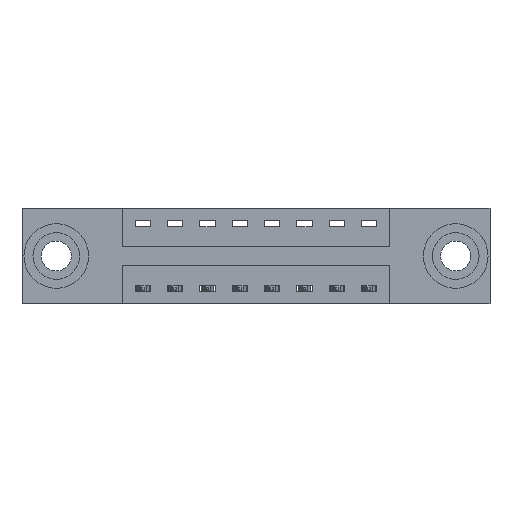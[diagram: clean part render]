
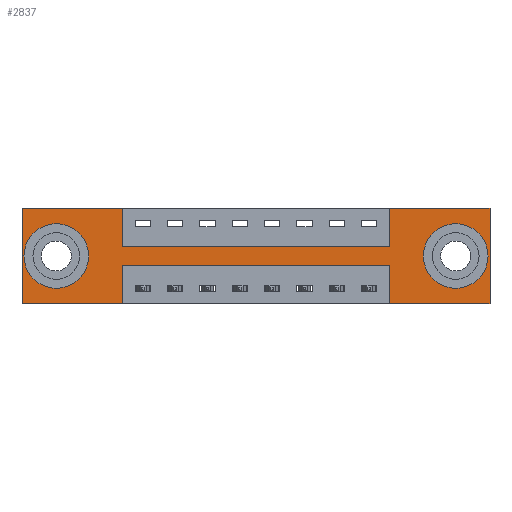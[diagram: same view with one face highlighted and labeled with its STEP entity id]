
A CAD part, front view. The second image highlights one B-rep face of the part: STEP entity #2837.
In plain terms, the highlighted planar face has unit normal (0, -1, 0).
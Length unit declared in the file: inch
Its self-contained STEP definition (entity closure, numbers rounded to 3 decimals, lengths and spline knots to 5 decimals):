
#114 = EDGE_CURVE ( 'NONE', #8169, #7383, #6678, .T. ) ;
#211 = CARTESIAN_POINT ( 'NONE',  ( 0., 0., -0.37 ) ) ;
#252 = LINE ( 'NONE', #2517, #8794 ) ;
#321 = CARTESIAN_POINT ( 'NONE',  ( 0.1325, 0., -0.185 ) ) ;
#346 = ORIENTED_EDGE ( 'NONE', *, *, #6904, .F. ) ;
#357 = CARTESIAN_POINT ( 'NONE',  ( 0., 0., -0.37 ) ) ;
#386 = CARTESIAN_POINT ( 'NONE',  ( 0., 0., 0. ) ) ;
#388 = ORIENTED_EDGE ( 'NONE', *, *, #9088, .F. ) ;
#441 = VERTEX_POINT ( 'NONE', #493 ) ;
#476 = VERTEX_POINT ( 'NONE', #3159 ) ;
#493 = CARTESIAN_POINT ( 'NONE',  ( 0.3875, 0., -0.37 ) ) ;
#588 = VECTOR ( 'NONE', #3738, 39.37008 ) ;
#693 = CARTESIAN_POINT ( 'NONE',  ( 0.3875, 0., -0.15 ) ) ;
#766 = CARTESIAN_POINT ( 'NONE',  ( 0., 0., 0. ) ) ;
#890 = CARTESIAN_POINT ( 'NONE',  ( 0.3875, 0., 0. ) ) ;
#983 = CARTESIAN_POINT ( 'NONE',  ( 0., 0., 0. ) ) ;
#1047 = DIRECTION ( 'NONE',  ( 0., 1., 0. ) ) ;
#1128 = VERTEX_POINT ( 'NONE', #7396 ) ;
#1168 = LINE ( 'NONE', #6201, #8599 ) ;
#1303 = AXIS2_PLACEMENT_3D ( 'NONE', #3767, #10361, #6446 ) ;
#1441 = EDGE_CURVE ( 'NONE', #8724, #7299, #5891, .T. ) ;
#1520 = ORIENTED_EDGE ( 'NONE', *, *, #4039, .F. ) ;
#1630 = DIRECTION ( 'NONE',  ( 1., 0., 0. ) ) ;
#1701 = VERTEX_POINT ( 'NONE', #5114 ) ;
#1726 = FACE_BOUND ( 'NONE', #5411, .T. ) ;
#1796 = EDGE_CURVE ( 'NONE', #476, #1128, #1168, .T. ) ;
#1880 = CARTESIAN_POINT ( 'NONE',  ( 1.4225, 0., -0.37 ) ) ;
#1891 = DIRECTION ( 'NONE',  ( 0., 0., -1. ) ) ;
#2003 = ORIENTED_EDGE ( 'NONE', *, *, #10641, .F. ) ;
#2126 = CARTESIAN_POINT ( 'NONE',  ( 0., 0., -0.37 ) ) ;
#2240 = EDGE_CURVE ( 'NONE', #7383, #8169, #3048, .T. ) ;
#2427 = ORIENTED_EDGE ( 'NONE', *, *, #6433, .F. ) ;
#2454 = CARTESIAN_POINT ( 'NONE',  ( 1.4225, 0., -0.37 ) ) ;
#2517 = CARTESIAN_POINT ( 'NONE',  ( 1.81, 0., 0. ) ) ;
#2661 = VERTEX_POINT ( 'NONE', #8579 ) ;
#2837 = ADVANCED_FACE ( 'NONE', ( #3336, #1726, #5143 ), #7646, .T. ) ;
#2914 = VERTEX_POINT ( 'NONE', #4494 ) ;
#2925 = CARTESIAN_POINT ( 'NONE',  ( 1.81, 0., -0.37 ) ) ;
#2957 = VECTOR ( 'NONE', #4897, 39.37008 ) ;
#3048 = CIRCLE ( 'NONE', #3399, 0.078 ) ;
#3065 = CIRCLE ( 'NONE', #5849, 0.078 ) ;
#3135 = EDGE_CURVE ( 'NONE', #5711, #2661, #3065, .T. ) ;
#3159 = CARTESIAN_POINT ( 'NONE',  ( 1.4225, 0., -0.22 ) ) ;
#3262 = LINE ( 'NONE', #2454, #5918 ) ;
#3263 = ORIENTED_EDGE ( 'NONE', *, *, #9256, .F. ) ;
#3296 = CARTESIAN_POINT ( 'NONE',  ( 1.6775, 0., -0.185 ) ) ;
#3336 = FACE_BOUND ( 'NONE', #6505, .T. ) ;
#3371 = ORIENTED_EDGE ( 'NONE', *, *, #6085, .F. ) ;
#3399 = AXIS2_PLACEMENT_3D ( 'NONE', #3296, #5803, #3412 ) ;
#3412 = DIRECTION ( 'NONE',  ( 0., 0., -1. ) ) ;
#3517 = DIRECTION ( 'NONE',  ( 1., 0., 0. ) ) ;
#3738 = DIRECTION ( 'NONE',  ( -1., 0., 0. ) ) ;
#3767 = CARTESIAN_POINT ( 'NONE',  ( 0.1325, 0., -0.185 ) ) ;
#3784 = DIRECTION ( 'NONE',  ( 1., 0., 0. ) ) ;
#3820 = LINE ( 'NONE', #9636, #6292 ) ;
#3974 = DIRECTION ( 'NONE',  ( 0., 0., 1. ) ) ;
#4039 = EDGE_CURVE ( 'NONE', #1128, #441, #9095, .T. ) ;
#4141 = DIRECTION ( 'NONE',  ( 0., 0., -1. ) ) ;
#4237 = DIRECTION ( 'NONE',  ( 0., 0., 1. ) ) ;
#4352 = VERTEX_POINT ( 'NONE', #7799 ) ;
#4494 = CARTESIAN_POINT ( 'NONE',  ( 0.3875, 0., -0.15 ) ) ;
#4515 = DIRECTION ( 'NONE',  ( -1., 0., 0. ) ) ;
#4550 = CARTESIAN_POINT ( 'NONE',  ( 1.6775, 0., -0.263 ) ) ;
#4602 = DIRECTION ( 'NONE',  ( -1., 0., 0. ) ) ;
#4876 = VECTOR ( 'NONE', #3784, 39.37008 ) ;
#4897 = DIRECTION ( 'NONE',  ( 0., 0., -1. ) ) ;
#5106 = VECTOR ( 'NONE', #1630, 39.37008 ) ;
#5114 = CARTESIAN_POINT ( 'NONE',  ( 1.81, 0., 0. ) ) ;
#5143 = FACE_OUTER_BOUND ( 'NONE', #7369, .T. ) ;
#5281 = LINE ( 'NONE', #386, #4876 ) ;
#5411 = EDGE_LOOP ( 'NONE', ( #9332, #7173 ) ) ;
#5568 = VERTEX_POINT ( 'NONE', #1880 ) ;
#5575 = DIRECTION ( 'NONE',  ( 0., 0., 1. ) ) ;
#5711 = VERTEX_POINT ( 'NONE', #8716 ) ;
#5755 = CARTESIAN_POINT ( 'NONE',  ( 0., 0., 0. ) ) ;
#5803 = DIRECTION ( 'NONE',  ( 0., 1., 0. ) ) ;
#5846 = DIRECTION ( 'NONE',  ( 0., 0., -1. ) ) ;
#5849 = AXIS2_PLACEMENT_3D ( 'NONE', #321, #1047, #6846 ) ;
#5891 = LINE ( 'NONE', #983, #10109 ) ;
#5918 = VECTOR ( 'NONE', #5575, 39.37008 ) ;
#6085 = EDGE_CURVE ( 'NONE', #7427, #5568, #7893, .T. ) ;
#6152 = EDGE_CURVE ( 'NONE', #7784, #1701, #5281, .T. ) ;
#6157 = AXIS2_PLACEMENT_3D ( 'NONE', #6772, #10035, #9517 ) ;
#6201 = CARTESIAN_POINT ( 'NONE',  ( 0.3875, 0., -0.22 ) ) ;
#6292 = VECTOR ( 'NONE', #3974, 39.37008 ) ;
#6433 = EDGE_CURVE ( 'NONE', #7299, #4352, #7658, .T. ) ;
#6441 = ORIENTED_EDGE ( 'NONE', *, *, #6152, .F. ) ;
#6445 = ORIENTED_EDGE ( 'NONE', *, *, #2240, .T. ) ;
#6446 = DIRECTION ( 'NONE',  ( 0., 0., 1. ) ) ;
#6505 = EDGE_LOOP ( 'NONE', ( #7525, #6445 ) ) ;
#6552 = CARTESIAN_POINT ( 'NONE',  ( 0.3875, 0., -0.37 ) ) ;
#6666 = CARTESIAN_POINT ( 'NONE',  ( 1.4225, 0., 0. ) ) ;
#6678 = CIRCLE ( 'NONE', #6157, 0.078 ) ;
#6709 = EDGE_CURVE ( 'NONE', #7972, #7784, #3820, .T. ) ;
#6772 = CARTESIAN_POINT ( 'NONE',  ( 1.6775, 0., -0.185 ) ) ;
#6846 = DIRECTION ( 'NONE',  ( 0., 0., 1. ) ) ;
#6888 = CARTESIAN_POINT ( 'NONE',  ( 0., 0., -0.37 ) ) ;
#6904 = EDGE_CURVE ( 'NONE', #4352, #2914, #8293, .T. ) ;
#7085 = LINE ( 'NONE', #357, #8394 ) ;
#7168 = CIRCLE ( 'NONE', #1303, 0.078 ) ;
#7173 = ORIENTED_EDGE ( 'NONE', *, *, #7208, .T. ) ;
#7208 = EDGE_CURVE ( 'NONE', #2661, #5711, #7168, .T. ) ;
#7216 = AXIS2_PLACEMENT_3D ( 'NONE', #6888, #8344, #1891 ) ;
#7299 = VERTEX_POINT ( 'NONE', #766 ) ;
#7369 = EDGE_LOOP ( 'NONE', ( #1520, #7918, #2003, #3371, #388, #6441, #9249, #7671, #346, #2427, #9571, #3263 ) ) ;
#7383 = VERTEX_POINT ( 'NONE', #4550 ) ;
#7396 = CARTESIAN_POINT ( 'NONE',  ( 0.3875, 0., -0.22 ) ) ;
#7427 = VERTEX_POINT ( 'NONE', #2925 ) ;
#7525 = ORIENTED_EDGE ( 'NONE', *, *, #114, .T. ) ;
#7572 = EDGE_CURVE ( 'NONE', #2914, #7972, #9071, .T. ) ;
#7646 = PLANE ( 'NONE',  #7216 ) ;
#7658 = LINE ( 'NONE', #5755, #8875 ) ;
#7671 = ORIENTED_EDGE ( 'NONE', *, *, #7572, .F. ) ;
#7784 = VERTEX_POINT ( 'NONE', #6666 ) ;
#7799 = CARTESIAN_POINT ( 'NONE',  ( 0.3875, 0., 0. ) ) ;
#7808 = CARTESIAN_POINT ( 'NONE',  ( 1.4225, 0., -0.15 ) ) ;
#7893 = LINE ( 'NONE', #2126, #588 ) ;
#7918 = ORIENTED_EDGE ( 'NONE', *, *, #1796, .F. ) ;
#7972 = VERTEX_POINT ( 'NONE', #7808 ) ;
#8169 = VERTEX_POINT ( 'NONE', #9037 ) ;
#8293 = LINE ( 'NONE', #890, #8889 ) ;
#8344 = DIRECTION ( 'NONE',  ( 0., -1., 0. ) ) ;
#8394 = VECTOR ( 'NONE', #4515, 39.37008 ) ;
#8579 = CARTESIAN_POINT ( 'NONE',  ( 0.1325, 0., -0.263 ) ) ;
#8599 = VECTOR ( 'NONE', #4602, 39.37008 ) ;
#8716 = CARTESIAN_POINT ( 'NONE',  ( 0.1325, 0., -0.107 ) ) ;
#8724 = VERTEX_POINT ( 'NONE', #211 ) ;
#8794 = VECTOR ( 'NONE', #5846, 39.37008 ) ;
#8875 = VECTOR ( 'NONE', #3517, 39.37008 ) ;
#8889 = VECTOR ( 'NONE', #4141, 39.37008 ) ;
#9037 = CARTESIAN_POINT ( 'NONE',  ( 1.6775, 0., -0.107 ) ) ;
#9071 = LINE ( 'NONE', #693, #5106 ) ;
#9088 = EDGE_CURVE ( 'NONE', #1701, #7427, #252, .T. ) ;
#9095 = LINE ( 'NONE', #6552, #2957 ) ;
#9249 = ORIENTED_EDGE ( 'NONE', *, *, #6709, .F. ) ;
#9256 = EDGE_CURVE ( 'NONE', #441, #8724, #7085, .T. ) ;
#9332 = ORIENTED_EDGE ( 'NONE', *, *, #3135, .T. ) ;
#9517 = DIRECTION ( 'NONE',  ( 0., 0., -1. ) ) ;
#9571 = ORIENTED_EDGE ( 'NONE', *, *, #1441, .F. ) ;
#9636 = CARTESIAN_POINT ( 'NONE',  ( 1.4225, 0., 0. ) ) ;
#10035 = DIRECTION ( 'NONE',  ( 0., 1., 0. ) ) ;
#10109 = VECTOR ( 'NONE', #4237, 39.37008 ) ;
#10361 = DIRECTION ( 'NONE',  ( 0., 1., 0. ) ) ;
#10641 = EDGE_CURVE ( 'NONE', #5568, #476, #3262, .T. ) ;
